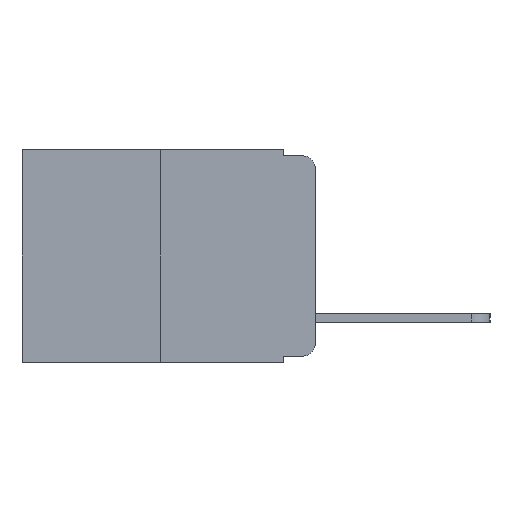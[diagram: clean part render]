
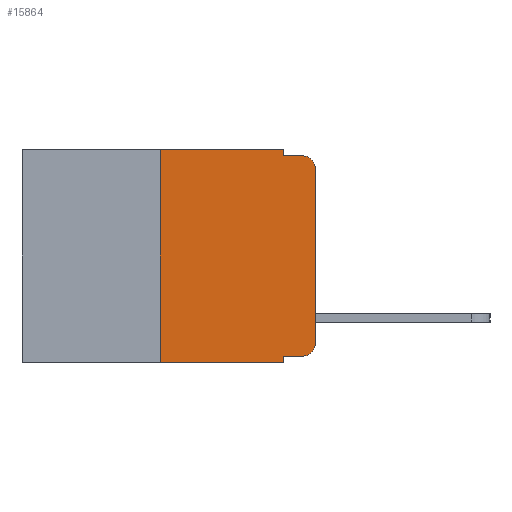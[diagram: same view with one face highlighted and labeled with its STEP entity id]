
A CAD part, left-side view. The second image highlights one B-rep face of the part: STEP entity #15864.
In plain terms, the highlighted planar face has unit normal (-1, 0, 0).
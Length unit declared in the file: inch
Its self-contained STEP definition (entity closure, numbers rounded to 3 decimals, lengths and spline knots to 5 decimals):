
#143 = ORIENTED_EDGE ( 'NONE', *, *, #12190, .F. ) ;
#232 = ORIENTED_EDGE ( 'NONE', *, *, #20031, .F. ) ;
#366 = ORIENTED_EDGE ( 'NONE', *, *, #10769, .T. ) ;
#756 = VERTEX_POINT ( 'NONE', #19013 ) ;
#954 = CARTESIAN_POINT ( 'NONE',  ( 0., 0.051, 0. ) ) ;
#1414 = CARTESIAN_POINT ( 'NONE',  ( 0., 0.02, -0.333 ) ) ;
#1526 = AXIS2_PLACEMENT_3D ( 'NONE', #12222, #19936, #10703 ) ;
#1554 = VECTOR ( 'NONE', #3282, 39.37008 ) ;
#1682 = ORIENTED_EDGE ( 'NONE', *, *, #2929, .F. ) ;
#1726 = VECTOR ( 'NONE', #13463, 39.37008 ) ;
#1868 = ORIENTED_EDGE ( 'NONE', *, *, #14498, .F. ) ;
#2019 = LINE ( 'NONE', #7387, #8789 ) ;
#2021 = CARTESIAN_POINT ( 'NONE',  ( 0., 0.02, -0.313 ) ) ;
#2929 = EDGE_CURVE ( 'NONE', #19372, #12352, #2019, .T. ) ;
#2963 = LINE ( 'NONE', #11317, #18015 ) ;
#3161 = EDGE_CURVE ( 'NONE', #3596, #17335, #13252, .T. ) ;
#3282 = DIRECTION ( 'NONE',  ( 0., -1., 0. ) ) ;
#3555 = DIRECTION ( 'NONE',  ( 0., 0., 1. ) ) ;
#3583 = DIRECTION ( 'NONE',  ( 0., 0., -1. ) ) ;
#3596 = VERTEX_POINT ( 'NONE', #5879 ) ;
#3739 = LINE ( 'NONE', #16591, #11530 ) ;
#3813 = ORIENTED_EDGE ( 'NONE', *, *, #3161, .T. ) ;
#4158 = AXIS2_PLACEMENT_3D ( 'NONE', #2021, #12946, #3583 ) ;
#4792 = CARTESIAN_POINT ( 'NONE',  ( 0., 0.051, -0.333 ) ) ;
#4814 = CARTESIAN_POINT ( 'NONE',  ( 0., 0.473, -0.343 ) ) ;
#5329 = VECTOR ( 'NONE', #13177, 39.37008 ) ;
#5425 = CARTESIAN_POINT ( 'NONE',  ( 0., 0.051, -0.01 ) ) ;
#5549 = FACE_OUTER_BOUND ( 'NONE', #10904, .T. ) ;
#5676 = LINE ( 'NONE', #4814, #1554 ) ;
#5879 = CARTESIAN_POINT ( 'NONE',  ( 0., 0.051, -0.333 ) ) ;
#6491 = DIRECTION ( 'NONE',  ( -1., 0., 0. ) ) ;
#6494 = ORIENTED_EDGE ( 'NONE', *, *, #14049, .F. ) ;
#7066 = DIRECTION ( 'NONE',  ( 0., -1., 0. ) ) ;
#7240 = VERTEX_POINT ( 'NONE', #8215 ) ;
#7300 = VERTEX_POINT ( 'NONE', #19629 ) ;
#7387 = CARTESIAN_POINT ( 'NONE',  ( 0., 0.051, 0. ) ) ;
#7935 = CARTESIAN_POINT ( 'NONE',  ( 0., 0.02, -0.01 ) ) ;
#8215 = CARTESIAN_POINT ( 'NONE',  ( 0., 0.051, -0.343 ) ) ;
#8380 = CARTESIAN_POINT ( 'NONE',  ( 0., 0.051, 0. ) ) ;
#8789 = VECTOR ( 'NONE', #18263, 39.37008 ) ;
#9112 = PLANE ( 'NONE',  #1526 ) ;
#10703 = DIRECTION ( 'NONE',  ( 0., 0., -1. ) ) ;
#10769 = EDGE_CURVE ( 'NONE', #15342, #7240, #5676, .T. ) ;
#10904 = EDGE_LOOP ( 'NONE', ( #18330, #18525, #143, #1682, #1868, #232, #366, #6494, #3813, #18536 ) ) ;
#11317 = CARTESIAN_POINT ( 'NONE',  ( 0., 0.25, 0. ) ) ;
#11530 = VECTOR ( 'NONE', #13584, 39.37008 ) ;
#11932 = EDGE_CURVE ( 'NONE', #756, #12566, #12247, .T. ) ;
#12135 = CARTESIAN_POINT ( 'NONE',  ( 0., 0.051, -0.01 ) ) ;
#12190 = EDGE_CURVE ( 'NONE', #12352, #12566, #12495, .T. ) ;
#12222 = CARTESIAN_POINT ( 'NONE',  ( 0., 0.473, 0. ) ) ;
#12225 = VERTEX_POINT ( 'NONE', #16473 ) ;
#12247 = CIRCLE ( 'NONE', #12319, 0.02 ) ;
#12319 = AXIS2_PLACEMENT_3D ( 'NONE', #15826, #6491, #17360 ) ;
#12352 = VERTEX_POINT ( 'NONE', #12135 ) ;
#12495 = LINE ( 'NONE', #5425, #16113 ) ;
#12566 = VERTEX_POINT ( 'NONE', #7935 ) ;
#12625 = DIRECTION ( 'NONE',  ( 0., -1., 0. ) ) ;
#12946 = DIRECTION ( 'NONE',  ( -1., 0., 0. ) ) ;
#13024 = CIRCLE ( 'NONE', #4158, 0.02 ) ;
#13177 = DIRECTION ( 'NONE',  ( 0., -1., 0. ) ) ;
#13252 = LINE ( 'NONE', #4792, #17334 ) ;
#13463 = DIRECTION ( 'NONE',  ( 0., 0., -1. ) ) ;
#13584 = DIRECTION ( 'NONE',  ( 0., 0., 1. ) ) ;
#13768 = CARTESIAN_POINT ( 'NONE',  ( 0., 0.25, -0.343 ) ) ;
#14049 = EDGE_CURVE ( 'NONE', #3596, #7240, #18249, .T. ) ;
#14498 = EDGE_CURVE ( 'NONE', #12225, #19372, #17751, .T. ) ;
#15342 = VERTEX_POINT ( 'NONE', #13768 ) ;
#15826 = CARTESIAN_POINT ( 'NONE',  ( 0., 0.02, -0.03 ) ) ;
#15864 = ADVANCED_FACE ( 'NONE', ( #5549 ), #9112, .F. ) ;
#16113 = VECTOR ( 'NONE', #7066, 39.37008 ) ;
#16473 = CARTESIAN_POINT ( 'NONE',  ( 0., 0.25, 0. ) ) ;
#16591 = CARTESIAN_POINT ( 'NONE',  ( 0., 0., 0. ) ) ;
#17334 = VECTOR ( 'NONE', #12625, 39.37008 ) ;
#17335 = VERTEX_POINT ( 'NONE', #1414 ) ;
#17360 = DIRECTION ( 'NONE',  ( 0., 0., -1. ) ) ;
#17735 = CARTESIAN_POINT ( 'NONE',  ( 0., 0.473, 0. ) ) ;
#17751 = LINE ( 'NONE', #17735, #5329 ) ;
#18015 = VECTOR ( 'NONE', #3555, 39.37008 ) ;
#18249 = LINE ( 'NONE', #954, #1726 ) ;
#18263 = DIRECTION ( 'NONE',  ( 0., 0., -1. ) ) ;
#18330 = ORIENTED_EDGE ( 'NONE', *, *, #18917, .T. ) ;
#18525 = ORIENTED_EDGE ( 'NONE', *, *, #11932, .T. ) ;
#18536 = ORIENTED_EDGE ( 'NONE', *, *, #19284, .T. ) ;
#18917 = EDGE_CURVE ( 'NONE', #7300, #756, #3739, .T. ) ;
#19013 = CARTESIAN_POINT ( 'NONE',  ( 0., 0., -0.03 ) ) ;
#19284 = EDGE_CURVE ( 'NONE', #17335, #7300, #13024, .T. ) ;
#19372 = VERTEX_POINT ( 'NONE', #8380 ) ;
#19629 = CARTESIAN_POINT ( 'NONE',  ( 0., 0., -0.313 ) ) ;
#19936 = DIRECTION ( 'NONE',  ( 1., 0., 0. ) ) ;
#20031 = EDGE_CURVE ( 'NONE', #15342, #12225, #2963, .T. ) ;
